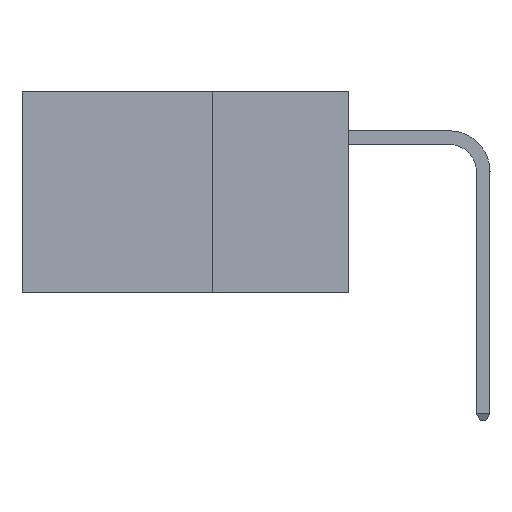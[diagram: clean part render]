
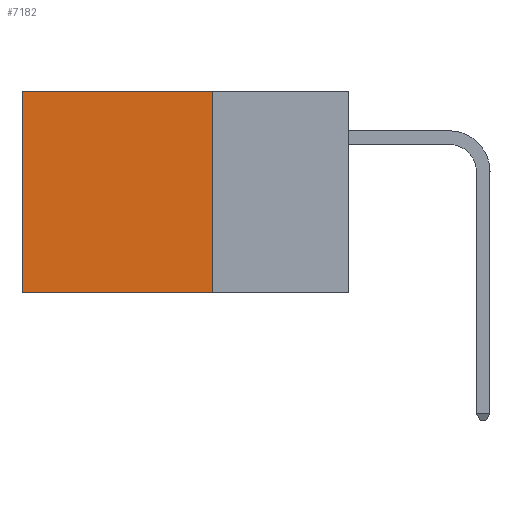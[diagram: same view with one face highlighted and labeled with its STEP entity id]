
A CAD part, left-side view. The second image highlights one B-rep face of the part: STEP entity #7182.
In plain terms, the highlighted planar face has unit normal (-1, 0, 0).
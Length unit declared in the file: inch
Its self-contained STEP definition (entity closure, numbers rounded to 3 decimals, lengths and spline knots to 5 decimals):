
#181 = VERTEX_POINT ( 'NONE', #9358 ) ;
#2843 = CARTESIAN_POINT ( 'NONE',  ( 0.2875, 0.25, -0.37 ) ) ;
#3068 = ORIENTED_EDGE ( 'NONE', *, *, #23833, .F. ) ;
#3797 = EDGE_CURVE ( 'NONE', #181, #12895, #31215, .T. ) ;
#7182 = ADVANCED_FACE ( 'NONE', ( #33906 ), #15969, .F. ) ;
#9288 = VECTOR ( 'NONE', #9386, 39.37008 ) ;
#9358 = CARTESIAN_POINT ( 'NONE',  ( 0.2875, 0.25, 0. ) ) ;
#9386 = DIRECTION ( 'NONE',  ( 0., 0., -1. ) ) ;
#10856 = LINE ( 'NONE', #23311, #18977 ) ;
#11004 = CARTESIAN_POINT ( 'NONE',  ( 0.2875, 0.6, 0. ) ) ;
#12895 = VERTEX_POINT ( 'NONE', #11004 ) ;
#13565 = EDGE_CURVE ( 'NONE', #12895, #40645, #17974, .T. ) ;
#15130 = ORIENTED_EDGE ( 'NONE', *, *, #3797, .T. ) ;
#15969 = PLANE ( 'NONE',  #21458 ) ;
#16108 = DIRECTION ( 'NONE',  ( 0., 0., -1. ) ) ;
#16462 = CARTESIAN_POINT ( 'NONE',  ( 0.2875, 0.6, -0.37 ) ) ;
#16956 = VECTOR ( 'NONE', #27138, 39.37008 ) ;
#17974 = LINE ( 'NONE', #22473, #9288 ) ;
#18977 = VECTOR ( 'NONE', #20172, 39.37008 ) ;
#20172 = DIRECTION ( 'NONE',  ( 0., 0., -1. ) ) ;
#20760 = VECTOR ( 'NONE', #25342, 39.37008 ) ;
#21304 = LINE ( 'NONE', #2843, #20760 ) ;
#21458 = AXIS2_PLACEMENT_3D ( 'NONE', #22608, #25738, #16108 ) ;
#22473 = CARTESIAN_POINT ( 'NONE',  ( 0.2875, 0.6, 0. ) ) ;
#22608 = CARTESIAN_POINT ( 'NONE',  ( 0.2875, 0.25, 0. ) ) ;
#23311 = CARTESIAN_POINT ( 'NONE',  ( 0.2875, 0.25, 0. ) ) ;
#23833 = EDGE_CURVE ( 'NONE', #181, #29784, #10856, .T. ) ;
#25342 = DIRECTION ( 'NONE',  ( 0., 1., 0. ) ) ;
#25738 = DIRECTION ( 'NONE',  ( 1., 0., 0. ) ) ;
#27138 = DIRECTION ( 'NONE',  ( 0., 1., 0. ) ) ;
#29784 = VERTEX_POINT ( 'NONE', #33788 ) ;
#31202 = EDGE_LOOP ( 'NONE', ( #33251, #35179, #3068, #15130 ) ) ;
#31215 = LINE ( 'NONE', #40061, #16956 ) ;
#31732 = EDGE_CURVE ( 'NONE', #29784, #40645, #21304, .T. ) ;
#33251 = ORIENTED_EDGE ( 'NONE', *, *, #13565, .T. ) ;
#33788 = CARTESIAN_POINT ( 'NONE',  ( 0.2875, 0.25, -0.37 ) ) ;
#33906 = FACE_OUTER_BOUND ( 'NONE', #31202, .T. ) ;
#35179 = ORIENTED_EDGE ( 'NONE', *, *, #31732, .F. ) ;
#40061 = CARTESIAN_POINT ( 'NONE',  ( 0.2875, 0.25, 0. ) ) ;
#40645 = VERTEX_POINT ( 'NONE', #16462 ) ;
